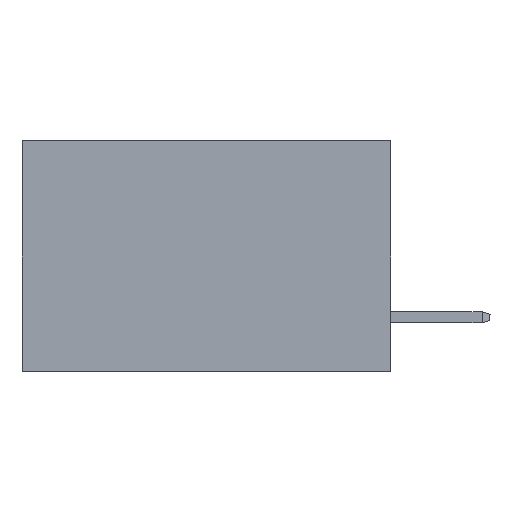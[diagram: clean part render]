
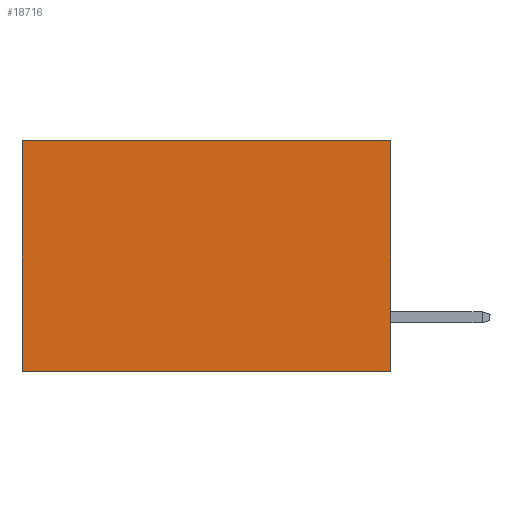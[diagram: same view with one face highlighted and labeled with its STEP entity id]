
A CAD part, left-side view. The second image highlights one B-rep face of the part: STEP entity #18716.
In plain terms, the highlighted planar face has unit normal (-1, 0, 0).
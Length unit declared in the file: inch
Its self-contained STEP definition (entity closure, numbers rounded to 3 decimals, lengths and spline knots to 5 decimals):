
#143 = CARTESIAN_POINT ( 'NONE',  ( 0.2875, 0.6, -0.375 ) ) ;
#688 = ORIENTED_EDGE ( 'NONE', *, *, #19453, .T. ) ;
#999 = CARTESIAN_POINT ( 'NONE',  ( 0.2875, 0.6, 0. ) ) ;
#1575 = DIRECTION ( 'NONE',  ( 0., 0., -1. ) ) ;
#2480 = ORIENTED_EDGE ( 'NONE', *, *, #18359, .F. ) ;
#3204 = DIRECTION ( 'NONE',  ( 0., 1., 0. ) ) ;
#3224 = DIRECTION ( 'NONE',  ( 0., 1., 0. ) ) ;
#4034 = FACE_OUTER_BOUND ( 'NONE', #20588, .T. ) ;
#4117 = CARTESIAN_POINT ( 'NONE',  ( 0.2875, 0.6, -0.375 ) ) ;
#4346 = EDGE_CURVE ( 'NONE', #19067, #16676, #16764, .T. ) ;
#4474 = AXIS2_PLACEMENT_3D ( 'NONE', #12594, #15689, #18956 ) ;
#5612 = CARTESIAN_POINT ( 'NONE',  ( 0.2875, 0., 0. ) ) ;
#6488 = VECTOR ( 'NONE', #6574, 39.37008 ) ;
#6574 = DIRECTION ( 'NONE',  ( 0., 0., -1. ) ) ;
#7201 = ORIENTED_EDGE ( 'NONE', *, *, #4346, .T. ) ;
#7219 = LINE ( 'NONE', #143, #6488 ) ;
#8404 = ORIENTED_EDGE ( 'NONE', *, *, #12060, .F. ) ;
#9407 = PLANE ( 'NONE',  #4474 ) ;
#11485 = VECTOR ( 'NONE', #3204, 39.37008 ) ;
#12060 = EDGE_CURVE ( 'NONE', #19067, #19202, #17093, .T. ) ;
#12443 = CARTESIAN_POINT ( 'NONE',  ( 0.2875, 0., -0.375 ) ) ;
#12594 = CARTESIAN_POINT ( 'NONE',  ( 0.2875, 0., -0.375 ) ) ;
#14969 = VECTOR ( 'NONE', #3224, 39.37008 ) ;
#15689 = DIRECTION ( 'NONE',  ( 1., 0., 0. ) ) ;
#15736 = LINE ( 'NONE', #17816, #11485 ) ;
#16676 = VERTEX_POINT ( 'NONE', #999 ) ;
#16764 = LINE ( 'NONE', #17550, #14969 ) ;
#17093 = LINE ( 'NONE', #20596, #20335 ) ;
#17550 = CARTESIAN_POINT ( 'NONE',  ( 0.2875, 0., 0. ) ) ;
#17816 = CARTESIAN_POINT ( 'NONE',  ( 0.2875, 0., -0.375 ) ) ;
#18078 = VERTEX_POINT ( 'NONE', #4117 ) ;
#18359 = EDGE_CURVE ( 'NONE', #19202, #18078, #15736, .T. ) ;
#18716 = ADVANCED_FACE ( 'NONE', ( #4034 ), #9407, .F. ) ;
#18956 = DIRECTION ( 'NONE',  ( 0., 0., -1. ) ) ;
#19067 = VERTEX_POINT ( 'NONE', #5612 ) ;
#19202 = VERTEX_POINT ( 'NONE', #12443 ) ;
#19453 = EDGE_CURVE ( 'NONE', #16676, #18078, #7219, .T. ) ;
#20335 = VECTOR ( 'NONE', #1575, 39.37008 ) ;
#20588 = EDGE_LOOP ( 'NONE', ( #688, #2480, #8404, #7201 ) ) ;
#20596 = CARTESIAN_POINT ( 'NONE',  ( 0.2875, 0., -0.375 ) ) ;
